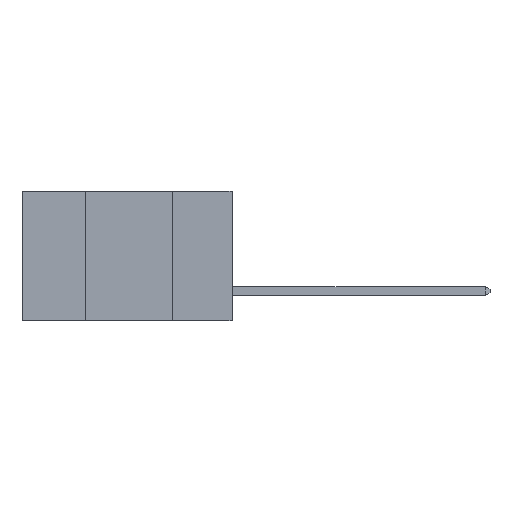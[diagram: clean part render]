
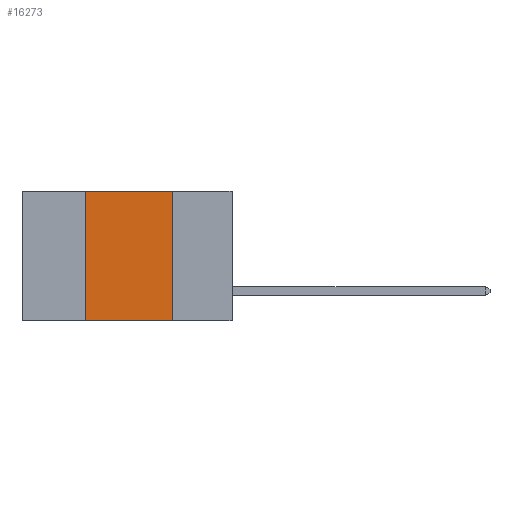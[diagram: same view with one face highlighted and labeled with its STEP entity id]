
A CAD part, left-side view. The second image highlights one B-rep face of the part: STEP entity #16273.
In plain terms, the highlighted planar face has unit normal (-1, 0, 0).
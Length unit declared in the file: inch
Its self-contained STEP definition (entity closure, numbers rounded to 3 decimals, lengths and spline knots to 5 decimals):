
#329 = ORIENTED_EDGE ( 'NONE', *, *, #16497, .F. ) ;
#481 = VERTEX_POINT ( 'NONE', #14626 ) ;
#1144 = DIRECTION ( 'NONE',  ( 0., -1., 0. ) ) ;
#1225 = EDGE_CURVE ( 'NONE', #13549, #4068, #22303, .T. ) ;
#1853 = CARTESIAN_POINT ( 'NONE',  ( 0., 0.6, 0. ) ) ;
#2332 = CARTESIAN_POINT ( 'NONE',  ( 0., 0.42, 0. ) ) ;
#2410 = ORIENTED_EDGE ( 'NONE', *, *, #1225, .F. ) ;
#3064 = AXIS2_PLACEMENT_3D ( 'NONE', #1853, #26122, #13066 ) ;
#3258 = CARTESIAN_POINT ( 'NONE',  ( 0., 0.17, 0. ) ) ;
#4002 = DIRECTION ( 'NONE',  ( 0., 0., 1. ) ) ;
#4068 = VERTEX_POINT ( 'NONE', #6590 ) ;
#6590 = CARTESIAN_POINT ( 'NONE',  ( 0., 0.42, 0. ) ) ;
#7819 = EDGE_CURVE ( 'NONE', #13549, #481, #27023, .T. ) ;
#9055 = VECTOR ( 'NONE', #23393, 39.37008 ) ;
#9106 = ORIENTED_EDGE ( 'NONE', *, *, #7819, .T. ) ;
#12193 = ORIENTED_EDGE ( 'NONE', *, *, #17612, .F. ) ;
#13066 = DIRECTION ( 'NONE',  ( 0., 0., -1. ) ) ;
#13549 = VERTEX_POINT ( 'NONE', #14346 ) ;
#14346 = CARTESIAN_POINT ( 'NONE',  ( 0., 0.42, -0.37 ) ) ;
#14626 = CARTESIAN_POINT ( 'NONE',  ( 0., 0.17, -0.37 ) ) ;
#15036 = EDGE_LOOP ( 'NONE', ( #329, #12193, #2410, #9106 ) ) ;
#15861 = VECTOR ( 'NONE', #4002, 39.37008 ) ;
#16012 = VERTEX_POINT ( 'NONE', #3258 ) ;
#16273 = ADVANCED_FACE ( 'NONE', ( #25302 ), #19538, .F. ) ;
#16497 = EDGE_CURVE ( 'NONE', #16012, #481, #26464, .T. ) ;
#17612 = EDGE_CURVE ( 'NONE', #4068, #16012, #20645, .T. ) ;
#19538 = PLANE ( 'NONE',  #3064 ) ;
#20645 = LINE ( 'NONE', #20937, #27103 ) ;
#20937 = CARTESIAN_POINT ( 'NONE',  ( 0., 0.6, 0. ) ) ;
#21174 = CARTESIAN_POINT ( 'NONE',  ( 0., 0.17, 0. ) ) ;
#21213 = CARTESIAN_POINT ( 'NONE',  ( 0., 0.6, -0.37 ) ) ;
#22303 = LINE ( 'NONE', #2332, #15861 ) ;
#23393 = DIRECTION ( 'NONE',  ( 0., 0., -1. ) ) ;
#25302 = FACE_OUTER_BOUND ( 'NONE', #15036, .T. ) ;
#26122 = DIRECTION ( 'NONE',  ( 1., 0., 0. ) ) ;
#26367 = VECTOR ( 'NONE', #27764, 39.37008 ) ;
#26464 = LINE ( 'NONE', #21174, #9055 ) ;
#27023 = LINE ( 'NONE', #21213, #26367 ) ;
#27103 = VECTOR ( 'NONE', #1144, 39.37008 ) ;
#27764 = DIRECTION ( 'NONE',  ( 0., -1., 0. ) ) ;
